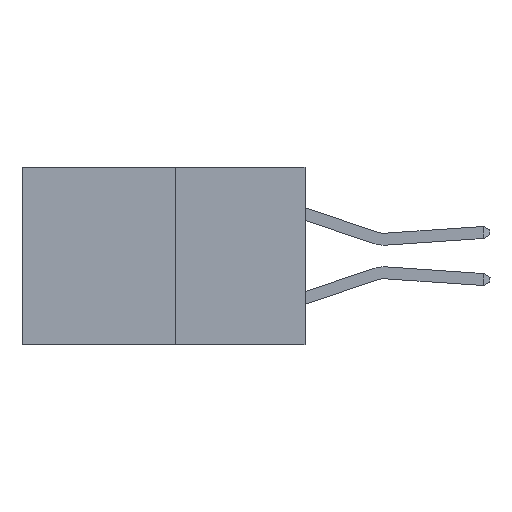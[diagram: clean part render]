
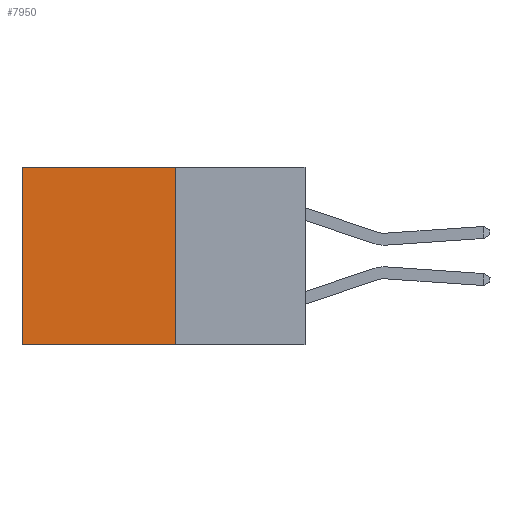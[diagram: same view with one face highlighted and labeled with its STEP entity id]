
A CAD part, left-side view. The second image highlights one B-rep face of the part: STEP entity #7950.
In plain terms, the highlighted planar face has unit normal (-1, 0, 0).
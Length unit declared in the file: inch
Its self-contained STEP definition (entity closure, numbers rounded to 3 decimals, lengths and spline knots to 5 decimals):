
#890 = EDGE_LOOP ( 'NONE', ( #24468, #20391, #12693, #15282 ) ) ;
#1046 = DIRECTION ( 'NONE',  ( 0., 0., -1. ) ) ;
#3047 = CARTESIAN_POINT ( 'NONE',  ( 0.277, 0.27, 0. ) ) ;
#3131 = VECTOR ( 'NONE', #15845, 39.37008 ) ;
#3238 = VECTOR ( 'NONE', #25834, 39.37008 ) ;
#3366 = PLANE ( 'NONE',  #25481 ) ;
#3502 = CARTESIAN_POINT ( 'NONE',  ( 0.277, 0.59, 0. ) ) ;
#4936 = EDGE_CURVE ( 'NONE', #23225, #15329, #20869, .T. ) ;
#5277 = DIRECTION ( 'NONE',  ( 0., 1., 0. ) ) ;
#7865 = CARTESIAN_POINT ( 'NONE',  ( 0.277, 0.27, -0.37 ) ) ;
#7950 = ADVANCED_FACE ( 'NONE', ( #25905 ), #3366, .F. ) ;
#8276 = CARTESIAN_POINT ( 'NONE',  ( 0.277, 0.27, 0. ) ) ;
#9442 = VECTOR ( 'NONE', #5277, 39.37008 ) ;
#10113 = DIRECTION ( 'NONE',  ( 0., 0., -1. ) ) ;
#12579 = CARTESIAN_POINT ( 'NONE',  ( 0.277, 0.27, -0.37 ) ) ;
#12693 = ORIENTED_EDGE ( 'NONE', *, *, #22158, .F. ) ;
#12842 = EDGE_CURVE ( 'NONE', #14323, #15329, #12996, .T. ) ;
#12996 = LINE ( 'NONE', #27596, #24097 ) ;
#13598 = CARTESIAN_POINT ( 'NONE',  ( 0.277, 0.27, -0.37 ) ) ;
#14323 = VERTEX_POINT ( 'NONE', #3502 ) ;
#15282 = ORIENTED_EDGE ( 'NONE', *, *, #21958, .T. ) ;
#15329 = VERTEX_POINT ( 'NONE', #21595 ) ;
#15845 = DIRECTION ( 'NONE',  ( 0., 1., 0. ) ) ;
#18058 = VERTEX_POINT ( 'NONE', #8276 ) ;
#20296 = LINE ( 'NONE', #12579, #3238 ) ;
#20378 = CARTESIAN_POINT ( 'NONE',  ( 0.277, 0.27, -0.37 ) ) ;
#20391 = ORIENTED_EDGE ( 'NONE', *, *, #4936, .F. ) ;
#20869 = LINE ( 'NONE', #13598, #3131 ) ;
#21216 = LINE ( 'NONE', #3047, #9442 ) ;
#21595 = CARTESIAN_POINT ( 'NONE',  ( 0.277, 0.59, -0.37 ) ) ;
#21958 = EDGE_CURVE ( 'NONE', #18058, #14323, #21216, .T. ) ;
#22158 = EDGE_CURVE ( 'NONE', #18058, #23225, #20296, .T. ) ;
#23225 = VERTEX_POINT ( 'NONE', #20378 ) ;
#23384 = DIRECTION ( 'NONE',  ( 1., 0., 0. ) ) ;
#24097 = VECTOR ( 'NONE', #1046, 39.37008 ) ;
#24468 = ORIENTED_EDGE ( 'NONE', *, *, #12842, .T. ) ;
#25481 = AXIS2_PLACEMENT_3D ( 'NONE', #7865, #23384, #10113 ) ;
#25834 = DIRECTION ( 'NONE',  ( 0., 0., -1. ) ) ;
#25905 = FACE_OUTER_BOUND ( 'NONE', #890, .T. ) ;
#27596 = CARTESIAN_POINT ( 'NONE',  ( 0.277, 0.59, -0.37 ) ) ;
